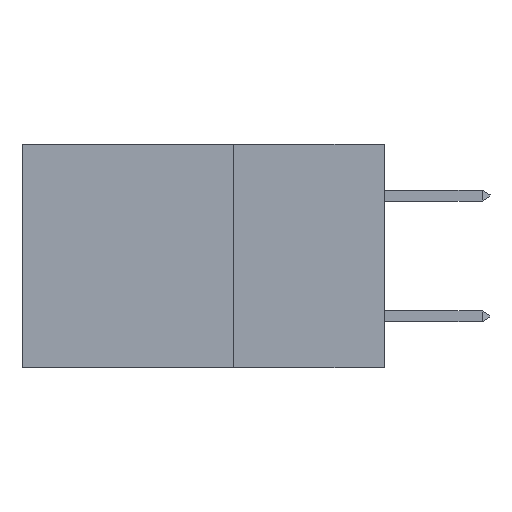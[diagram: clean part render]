
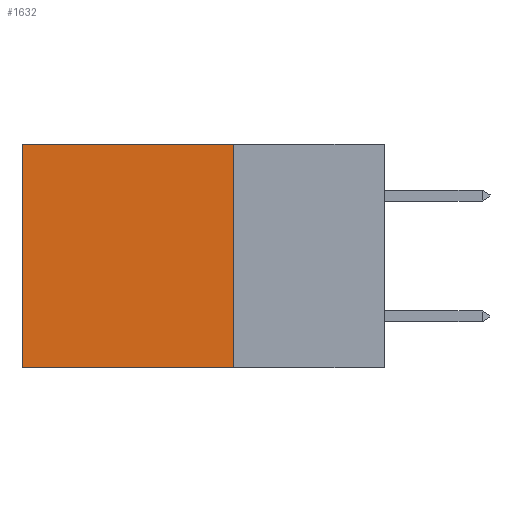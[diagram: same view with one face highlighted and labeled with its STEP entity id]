
A CAD part, left-side view. The second image highlights one B-rep face of the part: STEP entity #1632.
In plain terms, the highlighted planar face has unit normal (-1, 0, 0).
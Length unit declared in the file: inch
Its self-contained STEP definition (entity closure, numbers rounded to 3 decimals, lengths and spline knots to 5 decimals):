
#1632 = ADVANCED_FACE ( 'NONE', ( #2140 ), #6094, .F. ) ;
#2136 = DIRECTION ( 'NONE',  ( 0., 0., -1. ) ) ;
#2140 = FACE_OUTER_BOUND ( 'NONE', #8508, .T. ) ;
#5720 = EDGE_CURVE ( 'NONE', #12197, #27624, #25138, .T. ) ;
#6094 = PLANE ( 'NONE',  #15912 ) ;
#6541 = EDGE_CURVE ( 'NONE', #27624, #31326, #25070, .T. ) ;
#7385 = VECTOR ( 'NONE', #28732, 39.37008 ) ;
#8508 = EDGE_LOOP ( 'NONE', ( #29833, #32866, #8561, #32565 ) ) ;
#8561 = ORIENTED_EDGE ( 'NONE', *, *, #5720, .F. ) ;
#11526 = DIRECTION ( 'NONE',  ( 0., 0., -1. ) ) ;
#11773 = CARTESIAN_POINT ( 'NONE',  ( 0.2875, 0.25, 0. ) ) ;
#12197 = VERTEX_POINT ( 'NONE', #23543 ) ;
#14614 = CARTESIAN_POINT ( 'NONE',  ( 0.2875, 0.25, -0.37 ) ) ;
#15107 = CARTESIAN_POINT ( 'NONE',  ( 0.2875, 0.25, 0. ) ) ;
#15912 = AXIS2_PLACEMENT_3D ( 'NONE', #11773, #28185, #11526 ) ;
#16935 = VECTOR ( 'NONE', #2136, 39.37008 ) ;
#20348 = CARTESIAN_POINT ( 'NONE',  ( 0.2875, 0.6, 0. ) ) ;
#20607 = VECTOR ( 'NONE', #25694, 39.37008 ) ;
#21229 = CARTESIAN_POINT ( 'NONE',  ( 0.2875, 0.6, -0.37 ) ) ;
#23543 = CARTESIAN_POINT ( 'NONE',  ( 0.2875, 0.25, 0. ) ) ;
#23552 = CARTESIAN_POINT ( 'NONE',  ( 0.2875, 0.25, 0. ) ) ;
#24060 = CARTESIAN_POINT ( 'NONE',  ( 0.2875, 0.25, -0.37 ) ) ;
#25070 = LINE ( 'NONE', #14614, #7385 ) ;
#25138 = LINE ( 'NONE', #15107, #16935 ) ;
#25694 = DIRECTION ( 'NONE',  ( 0., 0., -1. ) ) ;
#27624 = VERTEX_POINT ( 'NONE', #24060 ) ;
#27923 = LINE ( 'NONE', #34286, #20607 ) ;
#28129 = EDGE_CURVE ( 'NONE', #32341, #31326, #27923, .T. ) ;
#28185 = DIRECTION ( 'NONE',  ( 1., 0., 0. ) ) ;
#28257 = EDGE_CURVE ( 'NONE', #12197, #32341, #32633, .T. ) ;
#28732 = DIRECTION ( 'NONE',  ( 0., 1., 0. ) ) ;
#29833 = ORIENTED_EDGE ( 'NONE', *, *, #28129, .T. ) ;
#30490 = VECTOR ( 'NONE', #34758, 39.37008 ) ;
#31326 = VERTEX_POINT ( 'NONE', #21229 ) ;
#32341 = VERTEX_POINT ( 'NONE', #20348 ) ;
#32565 = ORIENTED_EDGE ( 'NONE', *, *, #28257, .T. ) ;
#32633 = LINE ( 'NONE', #23552, #30490 ) ;
#32866 = ORIENTED_EDGE ( 'NONE', *, *, #6541, .F. ) ;
#34286 = CARTESIAN_POINT ( 'NONE',  ( 0.2875, 0.6, 0. ) ) ;
#34758 = DIRECTION ( 'NONE',  ( 0., 1., 0. ) ) ;
